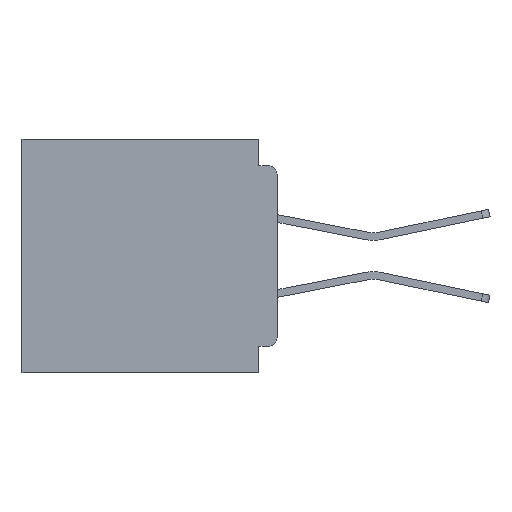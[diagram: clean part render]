
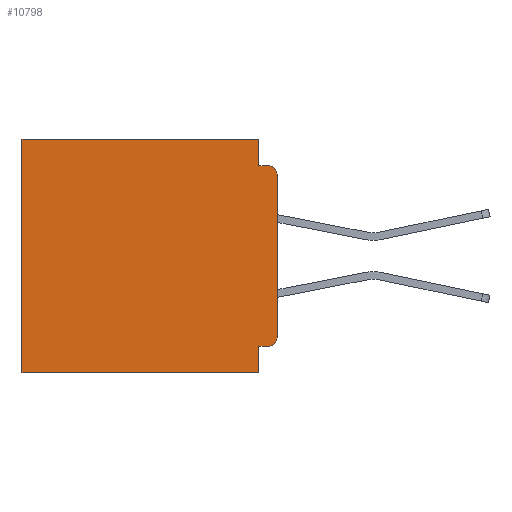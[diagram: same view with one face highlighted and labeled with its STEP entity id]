
A CAD part, left-side view. The second image highlights one B-rep face of the part: STEP entity #10798.
In plain terms, the highlighted planar face has unit normal (-1, 0, 0).
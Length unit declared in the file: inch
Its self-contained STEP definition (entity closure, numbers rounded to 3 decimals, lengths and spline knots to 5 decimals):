
#264 = VECTOR ( 'NONE', #7155, 39.37008 ) ;
#999 = DIRECTION ( 'NONE',  ( 0., 1., 0. ) ) ;
#1114 = CARTESIAN_POINT ( 'NONE',  ( 0.3, 0., -0.4 ) ) ;
#1388 = LINE ( 'NONE', #17740, #264 ) ;
#1977 = LINE ( 'NONE', #44364, #20966 ) ;
#2240 = VERTEX_POINT ( 'NONE', #5346 ) ;
#2709 = EDGE_CURVE ( 'NONE', #8390, #29847, #18075, .T. ) ;
#3130 = VERTEX_POINT ( 'NONE', #20787 ) ;
#3148 = AXIS2_PLACEMENT_3D ( 'NONE', #28709, #7279, #32308 ) ;
#3433 = EDGE_CURVE ( 'NONE', #2240, #21688, #9081, .T. ) ;
#3866 = VERTEX_POINT ( 'NONE', #12945 ) ;
#3907 = CARTESIAN_POINT ( 'NONE',  ( 0.3, 0.437, -0.4 ) ) ;
#4447 = VERTEX_POINT ( 'NONE', #45306 ) ;
#4902 = FACE_OUTER_BOUND ( 'NONE', #36355, .T. ) ;
#5346 = CARTESIAN_POINT ( 'NONE',  ( 0.3, 0., -0.06 ) ) ;
#6692 = LINE ( 'NONE', #8670, #24599 ) ;
#7155 = DIRECTION ( 'NONE',  ( 0., 0., -1. ) ) ;
#7238 = EDGE_CURVE ( 'NONE', #32692, #21688, #45872, .T. ) ;
#7279 = DIRECTION ( 'NONE',  ( -1., 0., 0. ) ) ;
#7298 = CARTESIAN_POINT ( 'NONE',  ( 0.3, 0., -0.045 ) ) ;
#8390 = VERTEX_POINT ( 'NONE', #10648 ) ;
#8670 = CARTESIAN_POINT ( 'NONE',  ( 0.3, 0., -0.355 ) ) ;
#9081 = CIRCLE ( 'NONE', #29262, 0.015 ) ;
#9517 = EDGE_CURVE ( 'NONE', #3866, #32692, #13908, .T. ) ;
#10648 = CARTESIAN_POINT ( 'NONE',  ( 0.3, 0.031, -0.4 ) ) ;
#10798 = ADVANCED_FACE ( 'NONE', ( #4902 ), #35075, .F. ) ;
#11562 = ORIENTED_EDGE ( 'NONE', *, *, #44301, .T. ) ;
#12250 = DIRECTION ( 'NONE',  ( 0., 1., 0. ) ) ;
#12945 = CARTESIAN_POINT ( 'NONE',  ( 0.3, 0.031, 0. ) ) ;
#13378 = DIRECTION ( 'NONE',  ( 0., 1., 0. ) ) ;
#13908 = LINE ( 'NONE', #34833, #31830 ) ;
#14010 = LINE ( 'NONE', #43870, #31944 ) ;
#14081 = CARTESIAN_POINT ( 'NONE',  ( 0.3, 0.031, -0.045 ) ) ;
#14881 = VERTEX_POINT ( 'NONE', #43893 ) ;
#17134 = DIRECTION ( 'NONE',  ( -1., 0., 0. ) ) ;
#17403 = CARTESIAN_POINT ( 'NONE',  ( 0.3, 0.015, -0.045 ) ) ;
#17740 = CARTESIAN_POINT ( 'NONE',  ( 0.3, 0., -0.4 ) ) ;
#17803 = ORIENTED_EDGE ( 'NONE', *, *, #23374, .T. ) ;
#18075 = LINE ( 'NONE', #1114, #36061 ) ;
#18601 = LINE ( 'NONE', #34579, #46076 ) ;
#18866 = EDGE_CURVE ( 'NONE', #3866, #3130, #14010, .T. ) ;
#20759 = DIRECTION ( 'NONE',  ( 1., 0., 0. ) ) ;
#20787 = CARTESIAN_POINT ( 'NONE',  ( 0.3, 0.437, 0. ) ) ;
#20966 = VECTOR ( 'NONE', #22872, 39.37008 ) ;
#21070 = CIRCLE ( 'NONE', #3148, 0.015 ) ;
#21326 = AXIS2_PLACEMENT_3D ( 'NONE', #42247, #20759, #45841 ) ;
#21688 = VERTEX_POINT ( 'NONE', #17403 ) ;
#22000 = EDGE_CURVE ( 'NONE', #4447, #8390, #1977, .T. ) ;
#22757 = ORIENTED_EDGE ( 'NONE', *, *, #25200, .F. ) ;
#22872 = DIRECTION ( 'NONE',  ( 0., 0., -1. ) ) ;
#23374 = EDGE_CURVE ( 'NONE', #3130, #29847, #18601, .T. ) ;
#24599 = VECTOR ( 'NONE', #12250, 39.37008 ) ;
#25200 = EDGE_CURVE ( 'NONE', #41978, #4447, #6692, .T. ) ;
#26190 = ORIENTED_EDGE ( 'NONE', *, *, #2709, .F. ) ;
#26526 = CARTESIAN_POINT ( 'NONE',  ( 0.3, 0.015, -0.06 ) ) ;
#27955 = VECTOR ( 'NONE', #35964, 39.37008 ) ;
#28709 = CARTESIAN_POINT ( 'NONE',  ( 0.3, 0.015, -0.34 ) ) ;
#29262 = AXIS2_PLACEMENT_3D ( 'NONE', #26526, #17134, #30022 ) ;
#29847 = VERTEX_POINT ( 'NONE', #3907 ) ;
#29876 = ORIENTED_EDGE ( 'NONE', *, *, #9517, .F. ) ;
#30022 = DIRECTION ( 'NONE',  ( 0., 0., -1. ) ) ;
#31181 = DIRECTION ( 'NONE',  ( 0., 0., -1. ) ) ;
#31830 = VECTOR ( 'NONE', #31181, 39.37008 ) ;
#31944 = VECTOR ( 'NONE', #999, 39.37008 ) ;
#32225 = ORIENTED_EDGE ( 'NONE', *, *, #18866, .T. ) ;
#32308 = DIRECTION ( 'NONE',  ( 0., 0., -1. ) ) ;
#32692 = VERTEX_POINT ( 'NONE', #14081 ) ;
#33279 = CARTESIAN_POINT ( 'NONE',  ( 0.3, 0.015, -0.355 ) ) ;
#33643 = EDGE_CURVE ( 'NONE', #2240, #14881, #1388, .T. ) ;
#33726 = ORIENTED_EDGE ( 'NONE', *, *, #33643, .F. ) ;
#34404 = ORIENTED_EDGE ( 'NONE', *, *, #7238, .F. ) ;
#34579 = CARTESIAN_POINT ( 'NONE',  ( 0.3, 0.437, -0.4 ) ) ;
#34833 = CARTESIAN_POINT ( 'NONE',  ( 0.3, 0.031, 0. ) ) ;
#35075 = PLANE ( 'NONE',  #21326 ) ;
#35964 = DIRECTION ( 'NONE',  ( 0., -1., 0. ) ) ;
#36061 = VECTOR ( 'NONE', #13378, 39.37008 ) ;
#36355 = EDGE_LOOP ( 'NONE', ( #33726, #44042, #34404, #29876, #32225, #17803, #26190, #43954, #22757, #11562 ) ) ;
#38173 = DIRECTION ( 'NONE',  ( 0., 0., -1. ) ) ;
#41978 = VERTEX_POINT ( 'NONE', #33279 ) ;
#42247 = CARTESIAN_POINT ( 'NONE',  ( 0.3, 0., -0.4 ) ) ;
#43870 = CARTESIAN_POINT ( 'NONE',  ( 0.3, 0., 0. ) ) ;
#43893 = CARTESIAN_POINT ( 'NONE',  ( 0.3, 0., -0.34 ) ) ;
#43954 = ORIENTED_EDGE ( 'NONE', *, *, #22000, .F. ) ;
#44042 = ORIENTED_EDGE ( 'NONE', *, *, #3433, .T. ) ;
#44301 = EDGE_CURVE ( 'NONE', #41978, #14881, #21070, .T. ) ;
#44364 = CARTESIAN_POINT ( 'NONE',  ( 0.3, 0.031, -0.4 ) ) ;
#45306 = CARTESIAN_POINT ( 'NONE',  ( 0.3, 0.031, -0.355 ) ) ;
#45841 = DIRECTION ( 'NONE',  ( 0., 0., -1. ) ) ;
#45872 = LINE ( 'NONE', #7298, #27955 ) ;
#46076 = VECTOR ( 'NONE', #38173, 39.37008 ) ;
